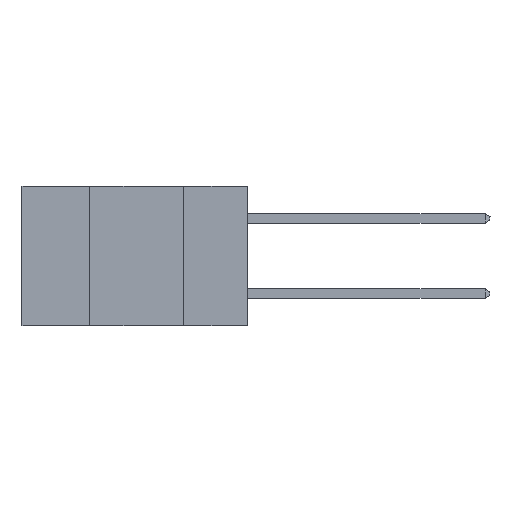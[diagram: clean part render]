
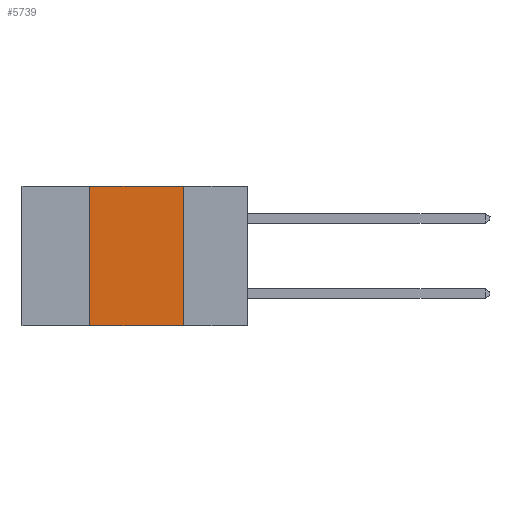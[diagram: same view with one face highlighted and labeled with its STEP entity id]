
A CAD part, left-side view. The second image highlights one B-rep face of the part: STEP entity #5739.
In plain terms, the highlighted planar face has unit normal (-1, 0, 0).
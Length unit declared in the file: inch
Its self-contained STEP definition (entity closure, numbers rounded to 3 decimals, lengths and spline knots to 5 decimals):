
#1059 = ORIENTED_EDGE ( 'NONE', *, *, #8338, .F. ) ;
#3153 = CARTESIAN_POINT ( 'NONE',  ( 0., 0.42, -0.37 ) ) ;
#3849 = FACE_OUTER_BOUND ( 'NONE', #23337, .T. ) ;
#3890 = DIRECTION ( 'NONE',  ( 0., 0., -1. ) ) ;
#4062 = DIRECTION ( 'NONE',  ( 0., -1., 0. ) ) ;
#4364 = VERTEX_POINT ( 'NONE', #19653 ) ;
#4444 = ORIENTED_EDGE ( 'NONE', *, *, #11800, .F. ) ;
#5007 = LINE ( 'NONE', #13750, #13502 ) ;
#5739 = ADVANCED_FACE ( 'NONE', ( #3849 ), #12942, .F. ) ;
#6038 = AXIS2_PLACEMENT_3D ( 'NONE', #15545, #6677, #7014 ) ;
#6070 = VECTOR ( 'NONE', #24378, 39.37008 ) ;
#6677 = DIRECTION ( 'NONE',  ( 1., 0., 0. ) ) ;
#7014 = DIRECTION ( 'NONE',  ( 0., 0., -1. ) ) ;
#8338 = EDGE_CURVE ( 'NONE', #23940, #20149, #15001, .T. ) ;
#9617 = LINE ( 'NONE', #15548, #24282 ) ;
#11800 = EDGE_CURVE ( 'NONE', #15608, #23940, #22100, .T. ) ;
#12570 = DIRECTION ( 'NONE',  ( 0., -1., 0. ) ) ;
#12942 = PLANE ( 'NONE',  #6038 ) ;
#13011 = CARTESIAN_POINT ( 'NONE',  ( 0., 0.42, 0. ) ) ;
#13080 = ORIENTED_EDGE ( 'NONE', *, *, #24405, .F. ) ;
#13502 = VECTOR ( 'NONE', #4062, 39.37008 ) ;
#13750 = CARTESIAN_POINT ( 'NONE',  ( 0., 0.6, -0.37 ) ) ;
#15001 = LINE ( 'NONE', #24521, #18946 ) ;
#15545 = CARTESIAN_POINT ( 'NONE',  ( 0., 0.6, 0. ) ) ;
#15548 = CARTESIAN_POINT ( 'NONE',  ( 0., 0.17, 0. ) ) ;
#15608 = VERTEX_POINT ( 'NONE', #3153 ) ;
#15728 = CARTESIAN_POINT ( 'NONE',  ( 0., 0.17, 0. ) ) ;
#18275 = EDGE_CURVE ( 'NONE', #15608, #4364, #5007, .T. ) ;
#18946 = VECTOR ( 'NONE', #12570, 39.37008 ) ;
#19605 = ORIENTED_EDGE ( 'NONE', *, *, #18275, .T. ) ;
#19653 = CARTESIAN_POINT ( 'NONE',  ( 0., 0.17, -0.37 ) ) ;
#19666 = CARTESIAN_POINT ( 'NONE',  ( 0., 0.42, 0. ) ) ;
#20149 = VERTEX_POINT ( 'NONE', #15728 ) ;
#22100 = LINE ( 'NONE', #13011, #6070 ) ;
#23337 = EDGE_LOOP ( 'NONE', ( #13080, #1059, #4444, #19605 ) ) ;
#23940 = VERTEX_POINT ( 'NONE', #19666 ) ;
#24282 = VECTOR ( 'NONE', #3890, 39.37008 ) ;
#24378 = DIRECTION ( 'NONE',  ( 0., 0., 1. ) ) ;
#24405 = EDGE_CURVE ( 'NONE', #20149, #4364, #9617, .T. ) ;
#24521 = CARTESIAN_POINT ( 'NONE',  ( 0., 0.6, 0. ) ) ;
